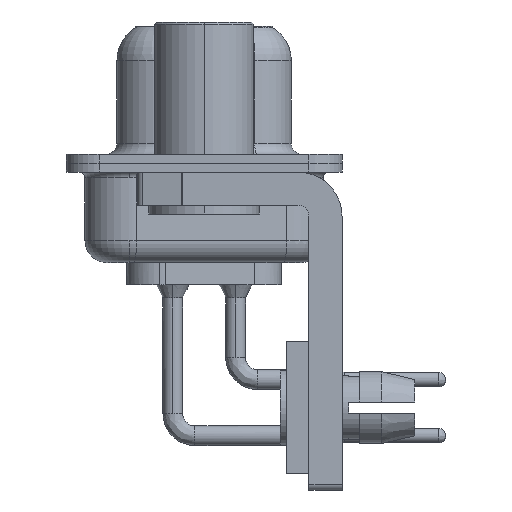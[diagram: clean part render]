
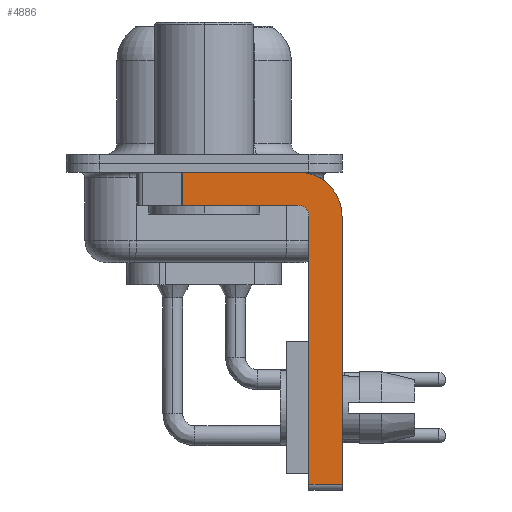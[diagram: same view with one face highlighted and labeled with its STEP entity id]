
A CAD part, left-side view. The second image highlights one B-rep face of the part: STEP entity #4886.
In plain terms, the highlighted planar face has unit normal (-1, 0, 0).
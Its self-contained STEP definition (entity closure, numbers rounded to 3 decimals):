
#696 = DIRECTION ( 'NONE',  ( 0., 0., -1. ) ) ;
#1042 = CARTESIAN_POINT ( 'NONE',  ( -2.9, -6.25, -2.4 ) ) ;
#1203 = DIRECTION ( 'NONE',  ( 0., 0., -1. ) ) ;
#1252 = CARTESIAN_POINT ( 'NONE',  ( -2.9, -4.25, -2.4 ) ) ;
#1936 = DIRECTION ( 'NONE',  ( -1., 0., 0. ) ) ;
#2167 = EDGE_CURVE ( 'NONE', #5975, #15426, #7197, .T. ) ;
#2661 = VECTOR ( 'NONE', #16094, 1000. ) ;
#2697 = FACE_OUTER_BOUND ( 'NONE', #22280, .T. ) ;
#3108 = CARTESIAN_POINT ( 'NONE',  ( -2.9, 3., -0.4 ) ) ;
#3225 = ORIENTED_EDGE ( 'NONE', *, *, #17279, .F. ) ;
#3964 = CARTESIAN_POINT ( 'NONE',  ( -2.9, -4.25, -1.9 ) ) ;
#4060 = CARTESIAN_POINT ( 'NONE',  ( -2.9, -4.75, -14.8 ) ) ;
#4460 = CARTESIAN_POINT ( 'NONE',  ( -2.9, -4.25, -1.9 ) ) ;
#4515 = EDGE_CURVE ( 'NONE', #15426, #15021, #26577, .T. ) ;
#4581 = ORIENTED_EDGE ( 'NONE', *, *, #18367, .F. ) ;
#4886 = ADVANCED_FACE ( 'NONE', ( #2697 ), #6704, .F. ) ;
#4896 = VECTOR ( 'NONE', #14602, 1000. ) ;
#5456 = ORIENTED_EDGE ( 'NONE', *, *, #11461, .T. ) ;
#5938 = CARTESIAN_POINT ( 'NONE',  ( -2.9, -4.75, -14.55 ) ) ;
#5975 = VERTEX_POINT ( 'NONE', #26937 ) ;
#6025 = CARTESIAN_POINT ( 'NONE',  ( -2.9, -6.25, -14.55 ) ) ;
#6329 = AXIS2_PLACEMENT_3D ( 'NONE', #1252, #1936, #9914 ) ;
#6448 = LINE ( 'NONE', #14348, #18533 ) ;
#6559 = ORIENTED_EDGE ( 'NONE', *, *, #24941, .F. ) ;
#6628 = VERTEX_POINT ( 'NONE', #23167 ) ;
#6704 = PLANE ( 'NONE',  #11885 ) ;
#7197 = CIRCLE ( 'NONE', #6329, 0.5 ) ;
#8716 = DIRECTION ( 'NONE',  ( 1., 0., 0. ) ) ;
#9914 = DIRECTION ( 'NONE',  ( 0., 0., 1. ) ) ;
#10373 = DIRECTION ( 'NONE',  ( 0., 1., 0. ) ) ;
#10629 = LINE ( 'NONE', #4060, #15741 ) ;
#11461 = EDGE_CURVE ( 'NONE', #6628, #15021, #6448, .T. ) ;
#11524 = VERTEX_POINT ( 'NONE', #6025 ) ;
#11881 = LINE ( 'NONE', #20934, #4896 ) ;
#11885 = AXIS2_PLACEMENT_3D ( 'NONE', #26494, #8716, #1203 ) ;
#12885 = VERTEX_POINT ( 'NONE', #5938 ) ;
#13536 = DIRECTION ( 'NONE',  ( 1., 0., 0. ) ) ;
#14213 = EDGE_CURVE ( 'NONE', #12885, #5975, #10629, .T. ) ;
#14348 = CARTESIAN_POINT ( 'NONE',  ( -2.9, 0.978, -1.9 ) ) ;
#14602 = DIRECTION ( 'NONE',  ( 0., -1., 0. ) ) ;
#14966 = ORIENTED_EDGE ( 'NONE', *, *, #15880, .T. ) ;
#15021 = VERTEX_POINT ( 'NONE', #21388 ) ;
#15194 = AXIS2_PLACEMENT_3D ( 'NONE', #26410, #13536, #696 ) ;
#15308 = ORIENTED_EDGE ( 'NONE', *, *, #14213, .F. ) ;
#15426 = VERTEX_POINT ( 'NONE', #3964 ) ;
#15741 = VECTOR ( 'NONE', #16947, 1000. ) ;
#15864 = VECTOR ( 'NONE', #10373, 1000. ) ;
#15880 = EDGE_CURVE ( 'NONE', #12885, #11524, #11881, .T. ) ;
#15929 = CIRCLE ( 'NONE', #15194, 2. ) ;
#16094 = DIRECTION ( 'NONE',  ( 0., 0., -1. ) ) ;
#16606 = VERTEX_POINT ( 'NONE', #19027 ) ;
#16947 = DIRECTION ( 'NONE',  ( 0., 0., 1. ) ) ;
#17148 = CARTESIAN_POINT ( 'NONE',  ( -2.9, -6.25, -2.4 ) ) ;
#17279 = EDGE_CURVE ( 'NONE', #24303, #11524, #19114, .T. ) ;
#18046 = ORIENTED_EDGE ( 'NONE', *, *, #2167, .F. ) ;
#18367 = EDGE_CURVE ( 'NONE', #6628, #16606, #25776, .T. ) ;
#18533 = VECTOR ( 'NONE', #22817, 1000. ) ;
#19027 = CARTESIAN_POINT ( 'NONE',  ( -2.9, -4.25, -0.4 ) ) ;
#19114 = LINE ( 'NONE', #1042, #2661 ) ;
#20032 = VECTOR ( 'NONE', #22410, 1000. ) ;
#20934 = CARTESIAN_POINT ( 'NONE',  ( -2.9, -4.25, -14.55 ) ) ;
#21374 = ORIENTED_EDGE ( 'NONE', *, *, #4515, .F. ) ;
#21388 = CARTESIAN_POINT ( 'NONE',  ( -2.9, 0.978, -1.9 ) ) ;
#22280 = EDGE_LOOP ( 'NONE', ( #4581, #5456, #21374, #18046, #15308, #14966, #3225, #6559 ) ) ;
#22410 = DIRECTION ( 'NONE',  ( 0., -1., 0. ) ) ;
#22817 = DIRECTION ( 'NONE',  ( 0., 0., -1. ) ) ;
#23167 = CARTESIAN_POINT ( 'NONE',  ( -2.9, 0.978, -0.4 ) ) ;
#24303 = VERTEX_POINT ( 'NONE', #17148 ) ;
#24941 = EDGE_CURVE ( 'NONE', #16606, #24303, #15929, .T. ) ;
#25776 = LINE ( 'NONE', #3108, #20032 ) ;
#26410 = CARTESIAN_POINT ( 'NONE',  ( -2.9, -4.25, -2.4 ) ) ;
#26494 = CARTESIAN_POINT ( 'NONE',  ( -2.9, -4.25, -2.4 ) ) ;
#26577 = LINE ( 'NONE', #4460, #15864 ) ;
#26937 = CARTESIAN_POINT ( 'NONE',  ( -2.9, -4.75, -2.4 ) ) ;
